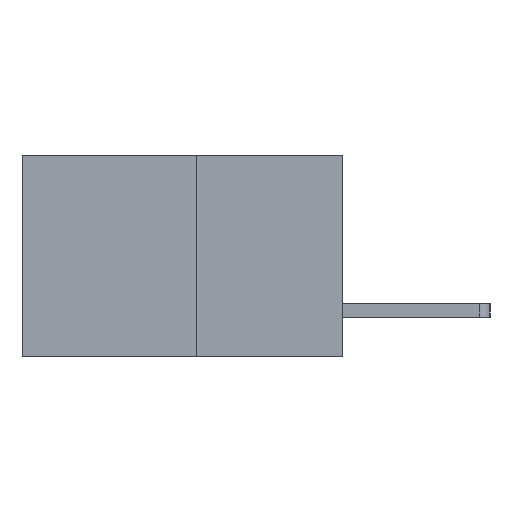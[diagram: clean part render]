
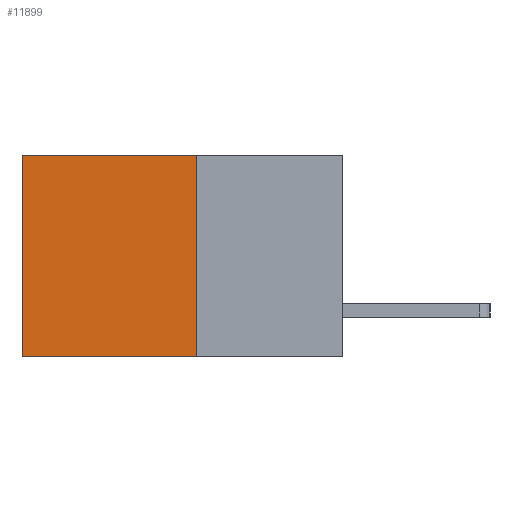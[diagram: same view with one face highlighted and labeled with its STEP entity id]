
A CAD part, left-side view. The second image highlights one B-rep face of the part: STEP entity #11899.
In plain terms, the highlighted planar face has unit normal (-1, 0, 0).
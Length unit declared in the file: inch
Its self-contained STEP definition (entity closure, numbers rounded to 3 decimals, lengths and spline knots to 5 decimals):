
#125 = ORIENTED_EDGE ( 'NONE', *, *, #2851, .T. ) ;
#400 = LINE ( 'NONE', #5514, #2650 ) ;
#553 = VERTEX_POINT ( 'NONE', #11308 ) ;
#870 = DIRECTION ( 'NONE',  ( 0., 0., -1. ) ) ;
#874 = CARTESIAN_POINT ( 'NONE',  ( 0.277, 0.27, -0.37 ) ) ;
#928 = CARTESIAN_POINT ( 'NONE',  ( 0.277, 0.27, -0.37 ) ) ;
#1879 = DIRECTION ( 'NONE',  ( 0., 0., -1. ) ) ;
#2244 = EDGE_CURVE ( 'NONE', #11233, #553, #11192, .T. ) ;
#2650 = VECTOR ( 'NONE', #5431, 39.37008 ) ;
#2851 = EDGE_CURVE ( 'NONE', #553, #3750, #400, .T. ) ;
#2941 = EDGE_LOOP ( 'NONE', ( #125, #7702, #10172, #5470 ) ) ;
#3288 = EDGE_CURVE ( 'NONE', #11233, #10686, #7673, .T. ) ;
#3750 = VERTEX_POINT ( 'NONE', #4870 ) ;
#3958 = CARTESIAN_POINT ( 'NONE',  ( 0.277, 0.27, -0.37 ) ) ;
#4624 = FACE_OUTER_BOUND ( 'NONE', #2941, .T. ) ;
#4870 = CARTESIAN_POINT ( 'NONE',  ( 0.277, 0.59, -0.37 ) ) ;
#5376 = CARTESIAN_POINT ( 'NONE',  ( 0.277, 0.27, -0.37 ) ) ;
#5431 = DIRECTION ( 'NONE',  ( 0., 0., -1. ) ) ;
#5470 = ORIENTED_EDGE ( 'NONE', *, *, #2244, .T. ) ;
#5514 = CARTESIAN_POINT ( 'NONE',  ( 0.277, 0.59, -0.37 ) ) ;
#5654 = PLANE ( 'NONE',  #11901 ) ;
#7558 = DIRECTION ( 'NONE',  ( 1., 0., 0. ) ) ;
#7673 = LINE ( 'NONE', #874, #7963 ) ;
#7702 = ORIENTED_EDGE ( 'NONE', *, *, #10411, .F. ) ;
#7963 = VECTOR ( 'NONE', #870, 39.37008 ) ;
#8693 = VECTOR ( 'NONE', #10369, 39.37008 ) ;
#9171 = DIRECTION ( 'NONE',  ( 0., 1., 0. ) ) ;
#9232 = VECTOR ( 'NONE', #9171, 39.37008 ) ;
#10172 = ORIENTED_EDGE ( 'NONE', *, *, #3288, .F. ) ;
#10369 = DIRECTION ( 'NONE',  ( 0., 1., 0. ) ) ;
#10411 = EDGE_CURVE ( 'NONE', #10686, #3750, #11726, .T. ) ;
#10495 = CARTESIAN_POINT ( 'NONE',  ( 0.277, 0.27, 0. ) ) ;
#10686 = VERTEX_POINT ( 'NONE', #3958 ) ;
#11192 = LINE ( 'NONE', #10495, #8693 ) ;
#11233 = VERTEX_POINT ( 'NONE', #11250 ) ;
#11250 = CARTESIAN_POINT ( 'NONE',  ( 0.277, 0.27, 0. ) ) ;
#11308 = CARTESIAN_POINT ( 'NONE',  ( 0.277, 0.59, 0. ) ) ;
#11726 = LINE ( 'NONE', #5376, #9232 ) ;
#11899 = ADVANCED_FACE ( 'NONE', ( #4624 ), #5654, .F. ) ;
#11901 = AXIS2_PLACEMENT_3D ( 'NONE', #928, #7558, #1879 ) ;
